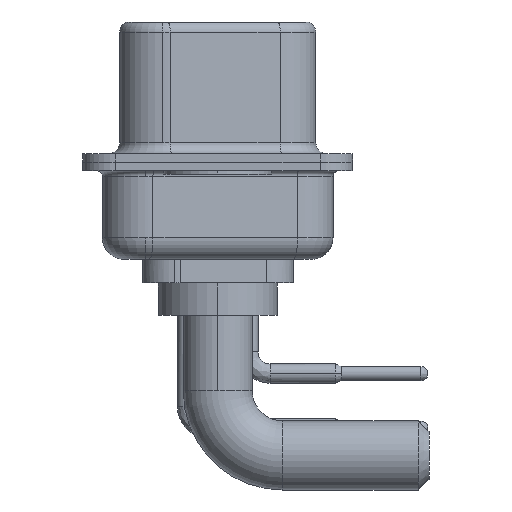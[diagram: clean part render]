
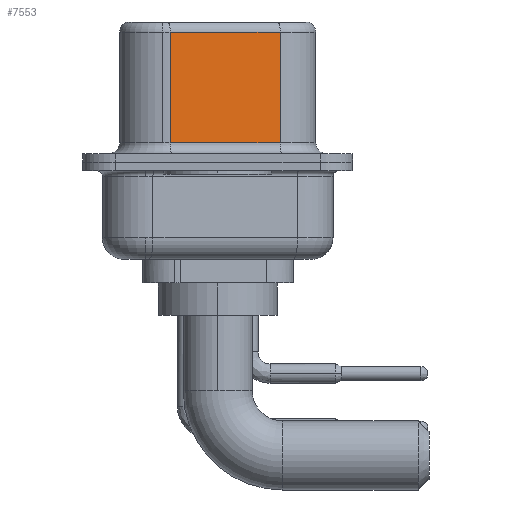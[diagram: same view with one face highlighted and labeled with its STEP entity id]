
A CAD part, left-side view. The second image highlights one B-rep face of the part: STEP entity #7553.
In plain terms, the highlighted planar face has unit normal (-0.985, -0.174, 0).
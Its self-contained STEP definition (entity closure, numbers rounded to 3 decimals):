
#40 = PLANE ( 'NONE',  #15159 ) ;
#748 = LINE ( 'NONE', #6062, #7711 ) ;
#960 = LINE ( 'NONE', #15430, #2799 ) ;
#1903 = DIRECTION ( 'NONE',  ( 0.985, 0.174, 0. ) ) ;
#2799 = VECTOR ( 'NONE', #6524, 1000. ) ;
#3653 = FACE_OUTER_BOUND ( 'NONE', #5509, .T. ) ;
#4259 = VERTEX_POINT ( 'NONE', #7389 ) ;
#5455 = ORIENTED_EDGE ( 'NONE', *, *, #7271, .T. ) ;
#5509 = EDGE_LOOP ( 'NONE', ( #19867, #8129, #5455, #8540 ) ) ;
#5619 = CARTESIAN_POINT ( 'NONE',  ( 4.58, -2.897, 0.9 ) ) ;
#5844 = VERTEX_POINT ( 'NONE', #5619 ) ;
#6062 = CARTESIAN_POINT ( 'NONE',  ( 3.68, 2.203, 6.52 ) ) ;
#6524 = DIRECTION ( 'NONE',  ( -0.174, 0.985, 0. ) ) ;
#6547 = VECTOR ( 'NONE', #18345, 1000. ) ;
#7271 = EDGE_CURVE ( 'NONE', #8713, #4259, #748, .T. ) ;
#7389 = CARTESIAN_POINT ( 'NONE',  ( 3.68, 2.203, 0.9 ) ) ;
#7553 = ADVANCED_FACE ( 'NONE', ( #3653 ), #40, .F. ) ;
#7711 = VECTOR ( 'NONE', #16862, 1000. ) ;
#7827 = LINE ( 'NONE', #10962, #11820 ) ;
#8129 = ORIENTED_EDGE ( 'NONE', *, *, #19289, .T. ) ;
#8540 = ORIENTED_EDGE ( 'NONE', *, *, #21553, .T. ) ;
#8713 = VERTEX_POINT ( 'NONE', #22544 ) ;
#10962 = CARTESIAN_POINT ( 'NONE',  ( 4.58, -2.897, 6.52 ) ) ;
#11820 = VECTOR ( 'NONE', #16653, 1000. ) ;
#13001 = CARTESIAN_POINT ( 'NONE',  ( 4.58, -2.897, 0.9 ) ) ;
#14278 = CARTESIAN_POINT ( 'NONE',  ( 4.58, -2.897, 6.52 ) ) ;
#15159 = AXIS2_PLACEMENT_3D ( 'NONE', #14278, #1903, #21014 ) ;
#15430 = CARTESIAN_POINT ( 'NONE',  ( 4.58, -2.897, 6.02 ) ) ;
#15684 = EDGE_CURVE ( 'NONE', #19610, #5844, #7827, .T. ) ;
#16653 = DIRECTION ( 'NONE',  ( 0., 0., -1. ) ) ;
#16862 = DIRECTION ( 'NONE',  ( 0., 0., -1. ) ) ;
#18345 = DIRECTION ( 'NONE',  ( 0.174, -0.985, 0. ) ) ;
#18784 = CARTESIAN_POINT ( 'NONE',  ( 4.58, -2.897, 6.02 ) ) ;
#19289 = EDGE_CURVE ( 'NONE', #19610, #8713, #960, .T. ) ;
#19610 = VERTEX_POINT ( 'NONE', #18784 ) ;
#19867 = ORIENTED_EDGE ( 'NONE', *, *, #15684, .F. ) ;
#20182 = LINE ( 'NONE', #13001, #6547 ) ;
#21014 = DIRECTION ( 'NONE',  ( -0.174, 0.985, 0. ) ) ;
#21553 = EDGE_CURVE ( 'NONE', #4259, #5844, #20182, .T. ) ;
#22544 = CARTESIAN_POINT ( 'NONE',  ( 3.68, 2.203, 6.02 ) ) ;
